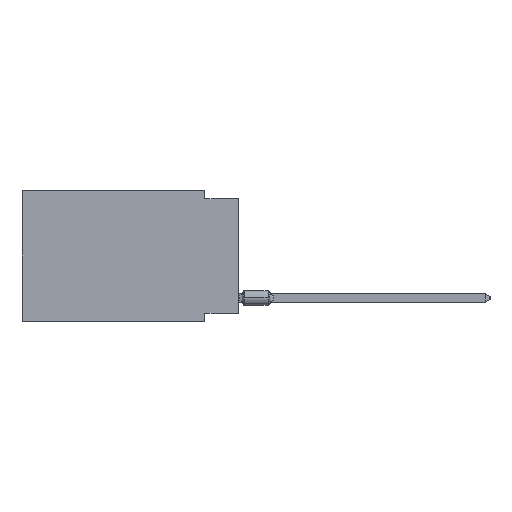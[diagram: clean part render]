
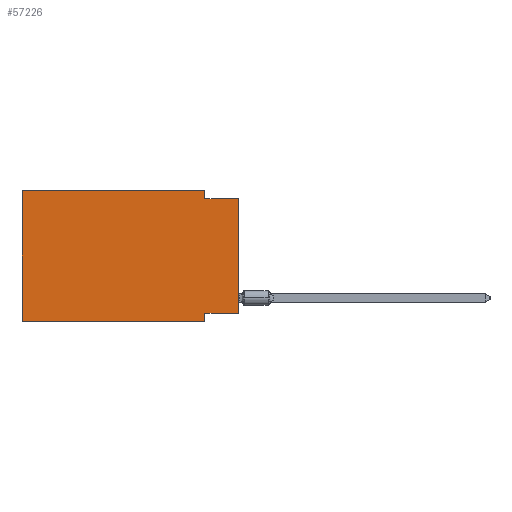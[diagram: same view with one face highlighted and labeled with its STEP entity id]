
A CAD part, left-side view. The second image highlights one B-rep face of the part: STEP entity #57226.
In plain terms, the highlighted planar face has unit normal (-1, 0, 0).
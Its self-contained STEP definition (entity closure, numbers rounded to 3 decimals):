
#1402 = VECTOR ( 'NONE', #17690, 1000. ) ;
#1521 = LINE ( 'NONE', #54156, #74364 ) ;
#3661 = VERTEX_POINT ( 'NONE', #82364 ) ;
#4860 = DIRECTION ( 'NONE',  ( 0., -1., 0. ) ) ;
#4997 = EDGE_CURVE ( 'NONE', #76628, #37589, #57295, .T. ) ;
#5790 = EDGE_CURVE ( 'NONE', #11522, #47729, #23870, .T. ) ;
#6245 = EDGE_LOOP ( 'NONE', ( #30529, #20352, #51249, #75989, #84476, #45771, #70469, #73917 ) ) ;
#6716 = EDGE_CURVE ( 'NONE', #3661, #76628, #32104, .T. ) ;
#6852 = FACE_OUTER_BOUND ( 'NONE', #6245, .T. ) ;
#8576 = EDGE_CURVE ( 'NONE', #37589, #11522, #37967, .T. ) ;
#9433 = VECTOR ( 'NONE', #26591, 1000. ) ;
#10127 = VECTOR ( 'NONE', #81391, 1000. ) ;
#10134 = CARTESIAN_POINT ( 'NONE',  ( 0., 2.54, -9.906 ) ) ;
#10196 = EDGE_CURVE ( 'NONE', #41489, #80873, #58827, .T. ) ;
#10718 = VECTOR ( 'NONE', #4860, 1000. ) ;
#11150 = DIRECTION ( 'NONE',  ( 0., -1., 0. ) ) ;
#11522 = VERTEX_POINT ( 'NONE', #23813 ) ;
#12372 = CARTESIAN_POINT ( 'NONE',  ( 0., 0., 0. ) ) ;
#13755 = DIRECTION ( 'NONE',  ( 1., 0., 0. ) ) ;
#17690 = DIRECTION ( 'NONE',  ( 0., 0., -1. ) ) ;
#18877 = CARTESIAN_POINT ( 'NONE',  ( 0., 16.383, 0. ) ) ;
#20352 = ORIENTED_EDGE ( 'NONE', *, *, #5790, .F. ) ;
#20414 = CARTESIAN_POINT ( 'NONE',  ( 0., 16.383, 0. ) ) ;
#23368 = CARTESIAN_POINT ( 'NONE',  ( 0., 2.54, -9.271 ) ) ;
#23813 = CARTESIAN_POINT ( 'NONE',  ( 0., 2.54, -0.635 ) ) ;
#23870 = LINE ( 'NONE', #62742, #10718 ) ;
#24767 = CARTESIAN_POINT ( 'NONE',  ( 0., 16.383, 0. ) ) ;
#26297 = VECTOR ( 'NONE', #77436, 1000. ) ;
#26591 = DIRECTION ( 'NONE',  ( 0., 0., 1. ) ) ;
#28383 = CARTESIAN_POINT ( 'NONE',  ( 0., 0., -9.271 ) ) ;
#29824 = CARTESIAN_POINT ( 'NONE',  ( 0., 2.54, 0. ) ) ;
#30529 = ORIENTED_EDGE ( 'NONE', *, *, #85384, .T. ) ;
#32104 = LINE ( 'NONE', #24767, #71446 ) ;
#34335 = LINE ( 'NONE', #42492, #10127 ) ;
#37589 = VERTEX_POINT ( 'NONE', #29824 ) ;
#37967 = LINE ( 'NONE', #56964, #1402 ) ;
#40095 = DIRECTION ( 'NONE',  ( 0., 0., -1. ) ) ;
#41489 = VERTEX_POINT ( 'NONE', #28383 ) ;
#42492 = CARTESIAN_POINT ( 'NONE',  ( 0., 2.54, -9.906 ) ) ;
#45771 = ORIENTED_EDGE ( 'NONE', *, *, #46477, .T. ) ;
#46451 = VECTOR ( 'NONE', #11150, 1000. ) ;
#46477 = EDGE_CURVE ( 'NONE', #3661, #57941, #1521, .T. ) ;
#47729 = VERTEX_POINT ( 'NONE', #83899 ) ;
#51249 = ORIENTED_EDGE ( 'NONE', *, *, #8576, .F. ) ;
#54156 = CARTESIAN_POINT ( 'NONE',  ( 0., 16.383, -9.906 ) ) ;
#56964 = CARTESIAN_POINT ( 'NONE',  ( 0., 2.54, 0. ) ) ;
#57226 = ADVANCED_FACE ( 'NONE', ( #6852 ), #59498, .F. ) ;
#57295 = LINE ( 'NONE', #18877, #46451 ) ;
#57400 = AXIS2_PLACEMENT_3D ( 'NONE', #72879, #13755, #40095 ) ;
#57941 = VERTEX_POINT ( 'NONE', #10134 ) ;
#58827 = LINE ( 'NONE', #85172, #26297 ) ;
#59498 = PLANE ( 'NONE',  #57400 ) ;
#62742 = CARTESIAN_POINT ( 'NONE',  ( 0., 0., -0.635 ) ) ;
#70469 = ORIENTED_EDGE ( 'NONE', *, *, #77344, .F. ) ;
#70940 = DIRECTION ( 'NONE',  ( 0., 0., 1. ) ) ;
#71446 = VECTOR ( 'NONE', #70940, 1000. ) ;
#72879 = CARTESIAN_POINT ( 'NONE',  ( 0., 16.383, 0. ) ) ;
#73917 = ORIENTED_EDGE ( 'NONE', *, *, #10196, .F. ) ;
#74364 = VECTOR ( 'NONE', #80517, 1000. ) ;
#75989 = ORIENTED_EDGE ( 'NONE', *, *, #4997, .F. ) ;
#76628 = VERTEX_POINT ( 'NONE', #20414 ) ;
#77344 = EDGE_CURVE ( 'NONE', #80873, #57941, #34335, .T. ) ;
#77436 = DIRECTION ( 'NONE',  ( 0., 1., 0. ) ) ;
#77971 = LINE ( 'NONE', #12372, #9433 ) ;
#80517 = DIRECTION ( 'NONE',  ( 0., -1., 0. ) ) ;
#80873 = VERTEX_POINT ( 'NONE', #23368 ) ;
#81391 = DIRECTION ( 'NONE',  ( 0., 0., -1. ) ) ;
#82364 = CARTESIAN_POINT ( 'NONE',  ( 0., 16.383, -9.906 ) ) ;
#83899 = CARTESIAN_POINT ( 'NONE',  ( 0., 0., -0.635 ) ) ;
#84476 = ORIENTED_EDGE ( 'NONE', *, *, #6716, .F. ) ;
#85172 = CARTESIAN_POINT ( 'NONE',  ( 0., 0., -9.271 ) ) ;
#85384 = EDGE_CURVE ( 'NONE', #41489, #47729, #77971, .T. ) ;
